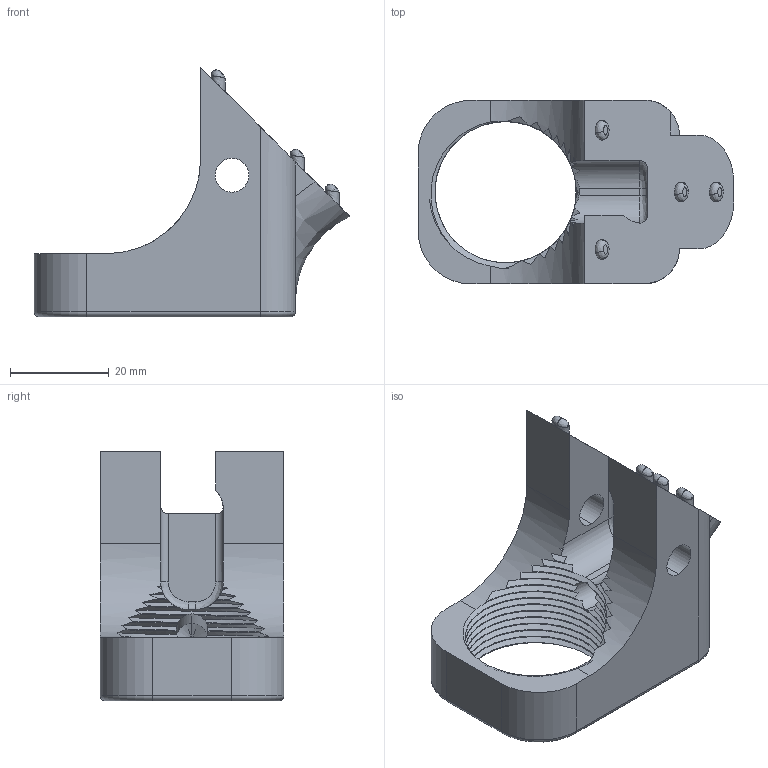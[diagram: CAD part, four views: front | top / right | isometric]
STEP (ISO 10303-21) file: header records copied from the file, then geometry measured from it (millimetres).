
FILE_DESCRIPTION (( 'STEP AP214' ), '1' );
FILE_NAME ('Vanilla_2.STEP', '2013-09-01T17:03:18', ( 'Asher' ), ( '' ), 'SwSTEP 2.0', 'SolidWorks 2013', '' );
FILE_SCHEMA (( 'AUTOMOTIVE_DESIGN' ));
Length unit declared in the file: millimetre
Products named in the file (1): Vanilla_2
Bounding box: 63.84 x 37.13 x 50.51 mm (x, y, z)
Volume: 32342.9 mm3; surface area: 12033.6 mm2
Topology: 1 solids, 1 shells, 133 faces, 369 edges, 238 vertices
Faces by surface type: cylinder 56, bspline 48, plane 21, cone 4, torus 4
Entity records: 32980 total; most frequent: CARTESIAN_POINT 30166, ORIENTED_EDGE 730, DIRECTION 397, EDGE_CURVE 365, VERTEX_POINT 238, AXIS2_PLACEMENT_3D 151, EDGE_LOOP 143, FACE_OUTER_BOUND 133
